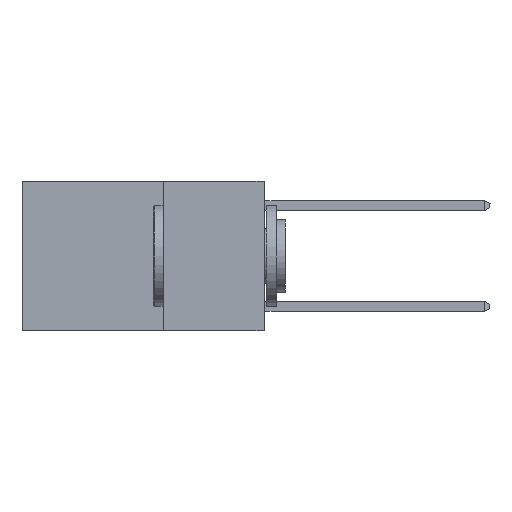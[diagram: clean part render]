
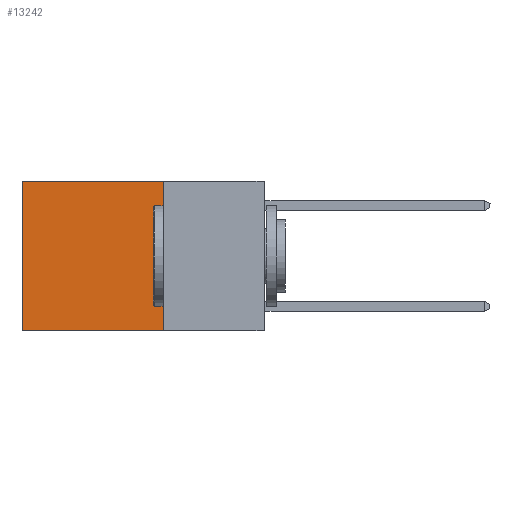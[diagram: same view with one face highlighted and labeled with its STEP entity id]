
A CAD part, left-side view. The second image highlights one B-rep face of the part: STEP entity #13242.
In plain terms, the highlighted planar face has unit normal (-1, 0, 0).
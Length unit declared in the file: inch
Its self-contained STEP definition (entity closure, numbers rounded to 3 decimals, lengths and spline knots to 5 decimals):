
#170 = CARTESIAN_POINT ( 'NONE',  ( 0.2625, 0.25, 0. ) ) ;
#176 = DIRECTION ( 'NONE',  ( 0., 0., -1. ) ) ;
#387 = VERTEX_POINT ( 'NONE', #1873 ) ;
#847 = CARTESIAN_POINT ( 'NONE',  ( 0.2625, 0.6, -0.37 ) ) ;
#893 = DIRECTION ( 'NONE',  ( 0., 0., -1. ) ) ;
#1109 = CARTESIAN_POINT ( 'NONE',  ( 0.2625, 0.25, 0. ) ) ;
#1144 = VECTOR ( 'NONE', #8519, 39.37008 ) ;
#1873 = CARTESIAN_POINT ( 'NONE',  ( 0.2625, 0.6, 0. ) ) ;
#2073 = VERTEX_POINT ( 'NONE', #847 ) ;
#2115 = VECTOR ( 'NONE', #176, 39.37008 ) ;
#2692 = FACE_OUTER_BOUND ( 'NONE', #16278, .T. ) ;
#2902 = PLANE ( 'NONE',  #12724 ) ;
#3969 = EDGE_CURVE ( 'NONE', #6964, #387, #4680, .T. ) ;
#4036 = DIRECTION ( 'NONE',  ( 0., 0., -1. ) ) ;
#4497 = ORIENTED_EDGE ( 'NONE', *, *, #5128, .T. ) ;
#4663 = CARTESIAN_POINT ( 'NONE',  ( 0.2625, 0.25, 0. ) ) ;
#4680 = LINE ( 'NONE', #170, #1144 ) ;
#5128 = EDGE_CURVE ( 'NONE', #387, #2073, #20887, .T. ) ;
#5952 = CARTESIAN_POINT ( 'NONE',  ( 0.2625, 0.25, -0.37 ) ) ;
#6964 = VERTEX_POINT ( 'NONE', #4663 ) ;
#7122 = LINE ( 'NONE', #8955, #20793 ) ;
#8519 = DIRECTION ( 'NONE',  ( 0., 1., 0. ) ) ;
#8566 = VECTOR ( 'NONE', #4036, 39.37008 ) ;
#8955 = CARTESIAN_POINT ( 'NONE',  ( 0.2625, 0.25, -0.37 ) ) ;
#11190 = VERTEX_POINT ( 'NONE', #5952 ) ;
#12443 = DIRECTION ( 'NONE',  ( 0., 1., 0. ) ) ;
#12724 = AXIS2_PLACEMENT_3D ( 'NONE', #1109, #17542, #893 ) ;
#13242 = ADVANCED_FACE ( 'NONE', ( #2692 ), #2902, .F. ) ;
#13588 = ORIENTED_EDGE ( 'NONE', *, *, #3969, .T. ) ;
#14387 = ORIENTED_EDGE ( 'NONE', *, *, #19139, .F. ) ;
#16278 = EDGE_LOOP ( 'NONE', ( #4497, #14387, #17371, #13588 ) ) ;
#17371 = ORIENTED_EDGE ( 'NONE', *, *, #17606, .F. ) ;
#17542 = DIRECTION ( 'NONE',  ( 1., 0., 0. ) ) ;
#17606 = EDGE_CURVE ( 'NONE', #6964, #11190, #18460, .T. ) ;
#18460 = LINE ( 'NONE', #19989, #2115 ) ;
#18816 = CARTESIAN_POINT ( 'NONE',  ( 0.2625, 0.6, 0. ) ) ;
#19139 = EDGE_CURVE ( 'NONE', #11190, #2073, #7122, .T. ) ;
#19989 = CARTESIAN_POINT ( 'NONE',  ( 0.2625, 0.25, 0. ) ) ;
#20793 = VECTOR ( 'NONE', #12443, 39.37008 ) ;
#20887 = LINE ( 'NONE', #18816, #8566 ) ;
